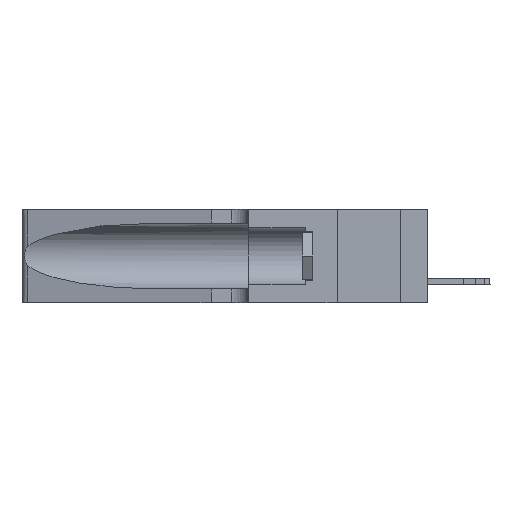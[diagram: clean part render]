
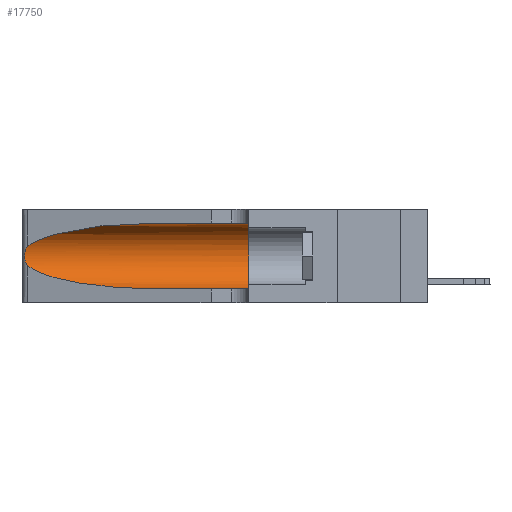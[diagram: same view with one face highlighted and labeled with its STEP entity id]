
A CAD part, left-side view. The second image highlights one B-rep face of the part: STEP entity #17750.
In plain terms, the highlighted cylindrical face has radius 3.308 mm (diameter 6.617 mm), a partial arc.
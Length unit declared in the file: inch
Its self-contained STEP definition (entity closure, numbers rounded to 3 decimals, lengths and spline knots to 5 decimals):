
#524 = DIRECTION ( 'NONE',  ( 0., 0., -1. ) ) ;
#947 = CYLINDRICAL_SURFACE ( 'NONE', #28229, 0.13025 ) ;
#1000 = CARTESIAN_POINT ( 'NONE',  ( 0.1305, 1.61858, 0.185 ) ) ;
#2205 = CIRCLE ( 'NONE', #20446, 0.13025 ) ;
#2966 = ORIENTED_EDGE ( 'NONE', *, *, #26123, .T. ) ;
#4774 = VERTEX_POINT ( 'NONE', #34297 ) ;
#5158 = CARTESIAN_POINT ( 'NONE',  ( 0.1305, 0.35, 0.185 ) ) ;
#5278 = CARTESIAN_POINT ( 'NONE',  ( 0.1305, 0.35, 0.05475 ) ) ;
#5678 = EDGE_CURVE ( 'NONE', #4774, #6689, #31708, .T. ) ;
#5702 = CARTESIAN_POINT ( 'NONE',  ( 0.1305, 1.61858, 0.05475 ) ) ;
#6041 = DIRECTION ( 'NONE',  ( 0., -1., 0. ) ) ;
#6166 = CARTESIAN_POINT ( 'NONE',  ( 0.2373, 1.15595, 0.08982 ) ) ;
#6285 = CARTESIAN_POINT ( 'NONE',  ( 0.26075, 1.23896, 0.178 ) ) ;
#6429 = EDGE_CURVE ( 'NONE', #28483, #22863, #18331, .T. ) ;
#6547 = ORIENTED_EDGE ( 'NONE', *, *, #6429, .T. ) ;
#6619 = CARTESIAN_POINT ( 'NONE',  ( 0.25639, 1.23186, 0.15144 ) ) ;
#6689 = VERTEX_POINT ( 'NONE', #5278 ) ;
#8774 = CARTESIAN_POINT ( 'NONE',  ( 0.1305, 0.35, 0.31525 ) ) ;
#9070 = CARTESIAN_POINT ( 'NONE',  ( 0.25856, 1.23593, 0.16098 ) ) ;
#9181 = CARTESIAN_POINT ( 'NONE',  ( 0.25789, 1.23486, 0.15765 ) ) ;
#9455 = CARTESIAN_POINT ( 'NONE',  ( 0.1305, 0.72297, 0.31525 ) ) ;
#9655 = EDGE_CURVE ( 'NONE', #14192, #6689, #2205, .T. ) ;
#9691 = CARTESIAN_POINT ( 'NONE',  ( 0.2373, 1.15595, 0.28018 ) ) ;
#11480 = CARTESIAN_POINT ( 'NONE',  ( 0.18966, 0.96281, 0.05475 ) ) ;
#11674 = CARTESIAN_POINT ( 'NONE',  ( 0.1305, 1.61858, 0.31525 ) ) ;
#13773 = CARTESIAN_POINT ( 'NONE',  ( 0.25487, 1.22718, 0.22369 ) ) ;
#14192 = VERTEX_POINT ( 'NONE', #8774 ) ;
#16568 = CARTESIAN_POINT ( 'NONE',  ( 0.25639, 1.23184, 0.21858 ) ) ;
#16615 = CARTESIAN_POINT ( 'NONE',  ( 0.1305, 0.72297, 0.31525 ) ) ;
#16685 = CARTESIAN_POINT ( 'NONE',  ( 0.25854, 1.2359, 0.20912 ) ) ;
#17110 = FACE_OUTER_BOUND ( 'NONE', #34394, .T. ) ;
#17287 = CARTESIAN_POINT ( 'NONE',  ( 0.25555, 1.22993, 0.14849 ) ) ;
#17750 = ADVANCED_FACE ( 'NONE', ( #17110 ), #947, .F. ) ;
#18191 = ORIENTED_EDGE ( 'NONE', *, *, #9655, .F. ) ;
#18331 = B_SPLINE_CURVE_WITH_KNOTS ( 'NONE', 3,
 ( #13773, #32544, #16568, #19237, #16685, #27895, #25090, #6285, #22506, #9070, #9181, #6619, #17287, #19926 ),
 .UNSPECIFIED., .F., .F.,
 ( 4, 2, 2, 2, 2, 2, 4 ),
 ( 0., 0.00027, 0.00053, 0.00107, 0.0016, 0.00187, 0.00214 ),
 .UNSPECIFIED. ) ;
#18900 = ORIENTED_EDGE ( 'NONE', *, *, #34217, .T. ) ;
#19145 = VECTOR ( 'NONE', #6041, 39.37008 ) ;
#19237 = CARTESIAN_POINT ( 'NONE',  ( 0.25787, 1.23484, 0.2124 ) ) ;
#19292 = DIRECTION ( 'NONE',  ( 0., -1., 0. ) ) ;
#19345 = CARTESIAN_POINT ( 'NONE',  ( 0.25487, 1.22718, 0.14631 ) ) ;
#19519 = VECTOR ( 'NONE', #22476, 39.37008 ) ;
#19706 = DIRECTION ( 'NONE',  ( 0., 0., 1. ) ) ;
#19926 = CARTESIAN_POINT ( 'NONE',  ( 0.25487, 1.22718, 0.14631 ) ) ;
#20446 = AXIS2_PLACEMENT_3D ( 'NONE', #5158, #34137, #19706 ) ;
#21385 = ORIENTED_EDGE ( 'NONE', *, *, #5678, .T. ) ;
#21978 = ORIENTED_EDGE ( 'NONE', *, *, #29026, .F. ) ;
#22476 = DIRECTION ( 'NONE',  ( 0., -1., 0. ) ) ;
#22506 = CARTESIAN_POINT ( 'NONE',  ( 0.26017, 1.23833, 0.17102 ) ) ;
#22863 = VERTEX_POINT ( 'NONE', #30602 ) ;
#25090 = CARTESIAN_POINT ( 'NONE',  ( 0.26075, 1.23896, 0.19203 ) ) ;
#26123 = EDGE_CURVE ( 'NONE', #31650, #28483, #34383, .T. ) ;
#26660 = LINE ( 'NONE', #11674, #19519 ) ;
#27895 = CARTESIAN_POINT ( 'NONE',  ( 0.26018, 1.23835, 0.19895 ) ) ;
#28188 = CARTESIAN_POINT ( 'NONE',  ( 0.18966, 0.96281, 0.31525 ) ) ;
#28229 = AXIS2_PLACEMENT_3D ( 'NONE', #1000, #19292, #524 ) ;
#28483 = VERTEX_POINT ( 'NONE', #32862 ) ;
#29026 = EDGE_CURVE ( 'NONE', #31650, #14192, #26660, .T. ) ;
#30091 = CARTESIAN_POINT ( 'NONE',  ( 0.1305, 0.72297, 0.05475 ) ) ;
#30602 = CARTESIAN_POINT ( 'NONE',  ( 0.25487, 1.22718, 0.14631 ) ) ;
#30718 =( BOUNDED_CURVE ( )  B_SPLINE_CURVE ( 3, ( #19345, #6166, #11480, #30091 ),
 .UNSPECIFIED., .F., .F. ) 
 B_SPLINE_CURVE_WITH_KNOTS ( ( 4, 4 ),
 ( 3.44316, 4.71239 ),
 .UNSPECIFIED. ) 
 CURVE ( )  GEOMETRIC_REPRESENTATION_ITEM ( )  RATIONAL_B_SPLINE_CURVE ( ( 1., 0.87, 0.87, 1. ) ) 
 REPRESENTATION_ITEM ( '' )  );
#31650 = VERTEX_POINT ( 'NONE', #16615 ) ;
#31708 = LINE ( 'NONE', #5702, #19145 ) ;
#32544 = CARTESIAN_POINT ( 'NONE',  ( 0.25555, 1.22994, 0.2215 ) ) ;
#32862 = CARTESIAN_POINT ( 'NONE',  ( 0.25487, 1.22718, 0.22369 ) ) ;
#33025 = CARTESIAN_POINT ( 'NONE',  ( 0.25487, 1.22718, 0.22369 ) ) ;
#34137 = DIRECTION ( 'NONE',  ( 0., 1., 0. ) ) ;
#34217 = EDGE_CURVE ( 'NONE', #22863, #4774, #30718, .T. ) ;
#34297 = CARTESIAN_POINT ( 'NONE',  ( 0.1305, 0.72297, 0.05475 ) ) ;
#34383 =( BOUNDED_CURVE ( )  B_SPLINE_CURVE ( 3, ( #9455, #28188, #9691, #33025 ),
 .UNSPECIFIED., .F., .T. ) 
 B_SPLINE_CURVE_WITH_KNOTS ( ( 4, 4 ),
 ( 1.5708, 2.84003 ),
 .UNSPECIFIED. ) 
 CURVE ( )  GEOMETRIC_REPRESENTATION_ITEM ( )  RATIONAL_B_SPLINE_CURVE ( ( 1., 0.87, 0.87, 1. ) ) 
 REPRESENTATION_ITEM ( '' )  );
#34394 = EDGE_LOOP ( 'NONE', ( #2966, #6547, #18900, #21385, #18191, #21978 ) ) ;
